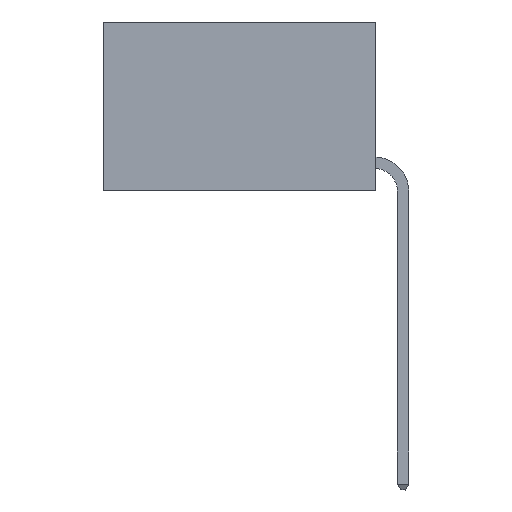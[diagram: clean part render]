
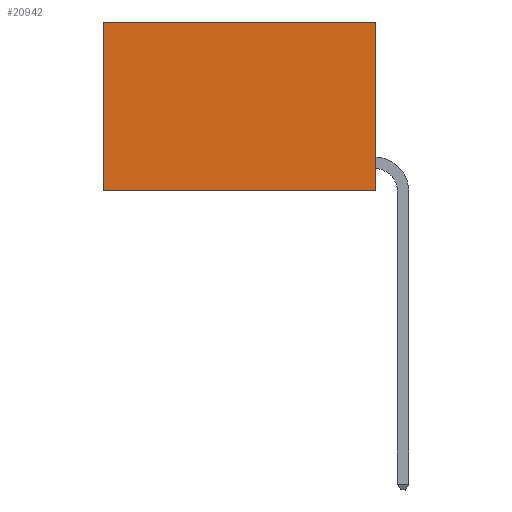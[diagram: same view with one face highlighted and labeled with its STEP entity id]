
A CAD part, left-side view. The second image highlights one B-rep face of the part: STEP entity #20942.
In plain terms, the highlighted planar face has unit normal (-1, 0, 0).
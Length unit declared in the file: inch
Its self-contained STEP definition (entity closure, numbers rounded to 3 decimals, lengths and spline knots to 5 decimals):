
#95 = CARTESIAN_POINT ( 'NONE',  ( 0.2625, 0., 0. ) ) ;
#1053 = LINE ( 'NONE', #19816, #21486 ) ;
#2138 = DIRECTION ( 'NONE',  ( 0., 0., -1. ) ) ;
#3019 = CARTESIAN_POINT ( 'NONE',  ( 0.2625, 0., 0. ) ) ;
#3923 = EDGE_CURVE ( 'NONE', #23595, #17479, #1053, .T. ) ;
#4090 = VECTOR ( 'NONE', #17244, 39.37008 ) ;
#4734 = EDGE_CURVE ( 'NONE', #8148, #23595, #17313, .T. ) ;
#7226 = VECTOR ( 'NONE', #15609, 39.37008 ) ;
#8148 = VERTEX_POINT ( 'NONE', #19945 ) ;
#8836 = ORIENTED_EDGE ( 'NONE', *, *, #22666, .T. ) ;
#11458 = CARTESIAN_POINT ( 'NONE',  ( 0.2625, 0., -0.37 ) ) ;
#11817 = VECTOR ( 'NONE', #26118, 39.37008 ) ;
#12602 = AXIS2_PLACEMENT_3D ( 'NONE', #95, #14349, #2138 ) ;
#13383 = CARTESIAN_POINT ( 'NONE',  ( 0.2625, 0.6, -0.37 ) ) ;
#13527 = CARTESIAN_POINT ( 'NONE',  ( 0.2625, 0.6, 0. ) ) ;
#14349 = DIRECTION ( 'NONE',  ( 1., 0., 0. ) ) ;
#15182 = EDGE_CURVE ( 'NONE', #8148, #17957, #25128, .T. ) ;
#15609 = DIRECTION ( 'NONE',  ( 0., 0., -1. ) ) ;
#15688 = DIRECTION ( 'NONE',  ( 0., 1., 0. ) ) ;
#17244 = DIRECTION ( 'NONE',  ( 0., 1., 0. ) ) ;
#17313 = LINE ( 'NONE', #20044, #11817 ) ;
#17479 = VERTEX_POINT ( 'NONE', #13383 ) ;
#17887 = EDGE_LOOP ( 'NONE', ( #8836, #24319, #23684, #23010 ) ) ;
#17957 = VERTEX_POINT ( 'NONE', #22901 ) ;
#18888 = FACE_OUTER_BOUND ( 'NONE', #17887, .T. ) ;
#19816 = CARTESIAN_POINT ( 'NONE',  ( 0.2625, 0., -0.37 ) ) ;
#19945 = CARTESIAN_POINT ( 'NONE',  ( 0.2625, 0., 0. ) ) ;
#20044 = CARTESIAN_POINT ( 'NONE',  ( 0.2625, 0., 0. ) ) ;
#20432 = PLANE ( 'NONE',  #12602 ) ;
#20942 = ADVANCED_FACE ( 'NONE', ( #18888 ), #20432, .F. ) ;
#21486 = VECTOR ( 'NONE', #15688, 39.37008 ) ;
#22666 = EDGE_CURVE ( 'NONE', #17957, #17479, #23516, .T. ) ;
#22901 = CARTESIAN_POINT ( 'NONE',  ( 0.2625, 0.6, 0. ) ) ;
#23010 = ORIENTED_EDGE ( 'NONE', *, *, #15182, .T. ) ;
#23516 = LINE ( 'NONE', #13527, #7226 ) ;
#23595 = VERTEX_POINT ( 'NONE', #11458 ) ;
#23684 = ORIENTED_EDGE ( 'NONE', *, *, #4734, .F. ) ;
#24319 = ORIENTED_EDGE ( 'NONE', *, *, #3923, .F. ) ;
#25128 = LINE ( 'NONE', #3019, #4090 ) ;
#26118 = DIRECTION ( 'NONE',  ( 0., 0., -1. ) ) ;
